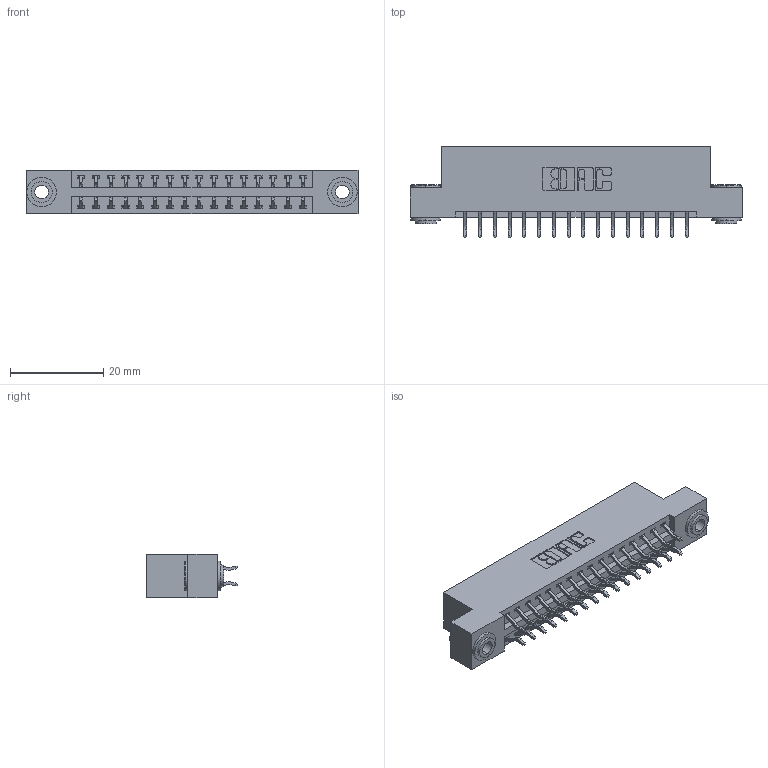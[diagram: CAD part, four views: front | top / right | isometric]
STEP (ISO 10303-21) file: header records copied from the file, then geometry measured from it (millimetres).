
FILE_DESCRIPTION (( 'STEP AP203' ), '1' );
FILE_NAME ('346-032-556-203.STEP', '2022-05-19T18:24:16', ( '' ), ( '' ), 'SwSTEP 2.0', 'SolidWorks 2020', '' );
FILE_SCHEMA (( 'CONFIG_CONTROL_DESIGN' ));
Length unit declared in the file: inch
Products named in the file (4): 345-250-002_345-250-002-102; 346-032-556-203; 345-292-001_556 Tail; 346 Part_Flush Mounting Lugs - 0.156 Dia-TH
Assembly tree (35 placements, depth 2):
  346-032-556-203
    346 Part_Flush Mounting Lugs - 0.156 Dia-TH
    345-292-001_556 Tail  x32
    345-250-002_345-250-002-102  x2
Bounding box: 71.37 x 19.57 x 9.4 mm (x, y, z)
Volume: 6757.9 mm3; surface area: 9099.6 mm2
Topology: 35 solids, 35 shells, 2030 faces, 5977 edges, 3938 vertices
Faces by surface type: plane 1348, cylinder 674, cone 8
Entity records: 15228 total; most frequent: CARTESIAN_POINT 2541, ORIENTED_EDGE 2454, DIRECTION 2309, EDGE_CURVE 1227, LINE 999, VECTOR 999, VERTEX_POINT 814, AXIS2_PLACEMENT_3D 655
